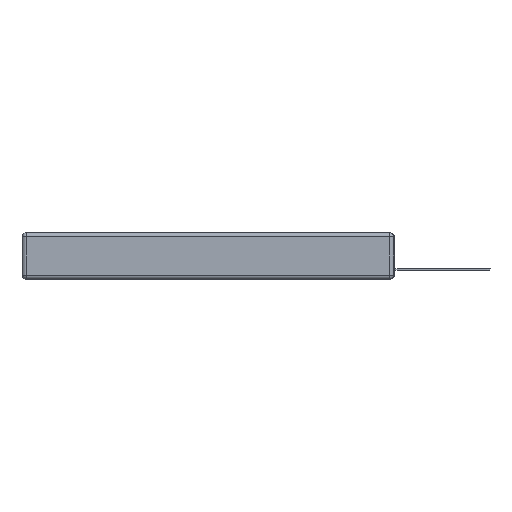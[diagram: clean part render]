
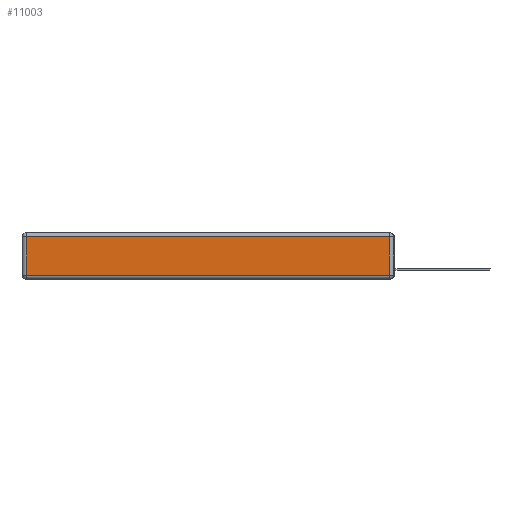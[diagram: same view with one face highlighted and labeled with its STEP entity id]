
A CAD part, left-side view. The second image highlights one B-rep face of the part: STEP entity #11003.
In plain terms, the highlighted planar face has unit normal (-1, 0, 0).
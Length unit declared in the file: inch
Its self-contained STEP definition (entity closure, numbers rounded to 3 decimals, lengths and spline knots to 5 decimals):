
#33 = DIRECTION ( 'NONE',  ( 0., -1., 0. ) ) ;
#591 = ORIENTED_EDGE ( 'NONE', *, *, #2821, .T. ) ;
#1146 = DIRECTION ( 'NONE',  ( -1., 0., 0. ) ) ;
#2040 = CARTESIAN_POINT ( 'NONE',  ( 0., 0.03, -0.03 ) ) ;
#2193 = LINE ( 'NONE', #2526, #10676 ) ;
#2526 = CARTESIAN_POINT ( 'NONE',  ( 0., 0., -0.313 ) ) ;
#2649 = VERTEX_POINT ( 'NONE', #9098 ) ;
#2821 = EDGE_CURVE ( 'NONE', #7834, #3057, #12825, .T. ) ;
#3057 = VERTEX_POINT ( 'NONE', #12347 ) ;
#4353 = CARTESIAN_POINT ( 'NONE',  ( 0., 2.72, -0.03 ) ) ;
#4388 = VERTEX_POINT ( 'NONE', #2040 ) ;
#4534 = ORIENTED_EDGE ( 'NONE', *, *, #12149, .T. ) ;
#5182 = LINE ( 'NONE', #12610, #13294 ) ;
#5695 = EDGE_LOOP ( 'NONE', ( #13131, #4534, #8566, #591 ) ) ;
#6144 = AXIS2_PLACEMENT_3D ( 'NONE', #12336, #1146, #12186 ) ;
#6169 = CARTESIAN_POINT ( 'NONE',  ( 0., 2.72, -0.343 ) ) ;
#6277 = EDGE_CURVE ( 'NONE', #4388, #7834, #7884, .T. ) ;
#7527 = FACE_OUTER_BOUND ( 'NONE', #5695, .T. ) ;
#7834 = VERTEX_POINT ( 'NONE', #4353 ) ;
#7884 = LINE ( 'NONE', #13760, #12524 ) ;
#8566 = ORIENTED_EDGE ( 'NONE', *, *, #6277, .T. ) ;
#8756 = VECTOR ( 'NONE', #14728, 39.37008 ) ;
#9098 = CARTESIAN_POINT ( 'NONE',  ( 0., 0.03, -0.313 ) ) ;
#10031 = EDGE_CURVE ( 'NONE', #3057, #2649, #2193, .T. ) ;
#10676 = VECTOR ( 'NONE', #33, 39.37008 ) ;
#11003 = ADVANCED_FACE ( 'NONE', ( #7527 ), #12134, .T. ) ;
#12134 = PLANE ( 'NONE',  #6144 ) ;
#12149 = EDGE_CURVE ( 'NONE', #2649, #4388, #5182, .T. ) ;
#12186 = DIRECTION ( 'NONE',  ( 0., 0., 1. ) ) ;
#12336 = CARTESIAN_POINT ( 'NONE',  ( 0., 0., -0.343 ) ) ;
#12347 = CARTESIAN_POINT ( 'NONE',  ( 0., 2.72, -0.313 ) ) ;
#12524 = VECTOR ( 'NONE', #14947, 39.37008 ) ;
#12610 = CARTESIAN_POINT ( 'NONE',  ( 0., 0.03, -0.343 ) ) ;
#12825 = LINE ( 'NONE', #6169, #8756 ) ;
#13131 = ORIENTED_EDGE ( 'NONE', *, *, #10031, .T. ) ;
#13294 = VECTOR ( 'NONE', #15311, 39.37008 ) ;
#13760 = CARTESIAN_POINT ( 'NONE',  ( 0., 2.75, -0.03 ) ) ;
#14728 = DIRECTION ( 'NONE',  ( 0., 0., -1. ) ) ;
#14947 = DIRECTION ( 'NONE',  ( 0., 1., 0. ) ) ;
#15311 = DIRECTION ( 'NONE',  ( 0., 0., 1. ) ) ;
